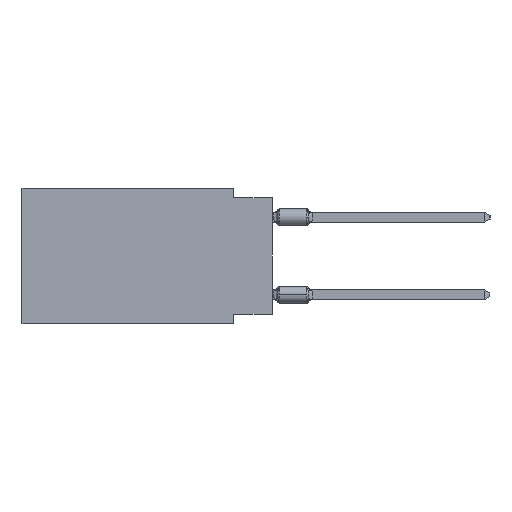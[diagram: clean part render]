
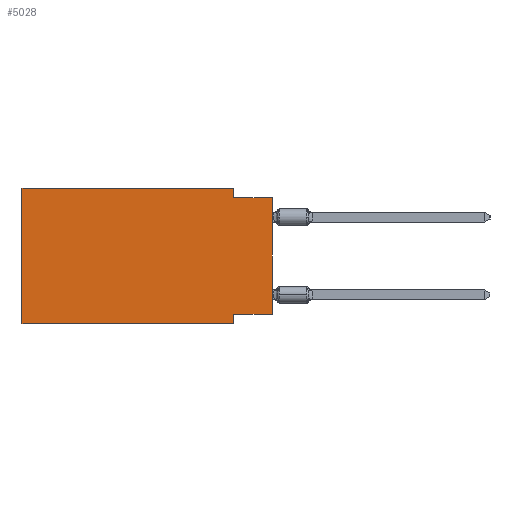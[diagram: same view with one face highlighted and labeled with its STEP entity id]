
A CAD part, left-side view. The second image highlights one B-rep face of the part: STEP entity #5028.
In plain terms, the highlighted planar face has unit normal (-1, 0, 0).
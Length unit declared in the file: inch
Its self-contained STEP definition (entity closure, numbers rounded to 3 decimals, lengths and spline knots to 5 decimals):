
#261 = DIRECTION ( 'NONE',  ( 0., -1., 0. ) ) ;
#508 = ORIENTED_EDGE ( 'NONE', *, *, #28338, .F. ) ;
#1469 = CARTESIAN_POINT ( 'NONE',  ( 0., 0.1, 0. ) ) ;
#1849 = AXIS2_PLACEMENT_3D ( 'NONE', #16052, #23807, #29257 ) ;
#3038 = ORIENTED_EDGE ( 'NONE', *, *, #13837, .T. ) ;
#3196 = LINE ( 'NONE', #21132, #12937 ) ;
#3567 = DIRECTION ( 'NONE',  ( 0., 0., 1. ) ) ;
#3634 = VECTOR ( 'NONE', #3567, 39.37008 ) ;
#4015 = VERTEX_POINT ( 'NONE', #17050 ) ;
#4470 = VECTOR ( 'NONE', #19000, 39.37008 ) ;
#4859 = VECTOR ( 'NONE', #8690, 39.37008 ) ;
#5028 = ADVANCED_FACE ( 'NONE', ( #29084 ), #23972, .F. ) ;
#5679 = CARTESIAN_POINT ( 'NONE',  ( 0., 0.645, -0.35 ) ) ;
#6104 = CARTESIAN_POINT ( 'NONE',  ( 0., 0.1, -0.35 ) ) ;
#7061 = EDGE_CURVE ( 'NONE', #13151, #31443, #3196, .T. ) ;
#7130 = DIRECTION ( 'NONE',  ( 0., 1., 0. ) ) ;
#7757 = EDGE_CURVE ( 'NONE', #9319, #26958, #9217, .T. ) ;
#8463 = ORIENTED_EDGE ( 'NONE', *, *, #7061, .T. ) ;
#8530 = LINE ( 'NONE', #16111, #4859 ) ;
#8581 = CARTESIAN_POINT ( 'NONE',  ( 0., 0., -0.325 ) ) ;
#8690 = DIRECTION ( 'NONE',  ( 0., -1., 0. ) ) ;
#9217 = LINE ( 'NONE', #24230, #27576 ) ;
#9319 = VERTEX_POINT ( 'NONE', #9963 ) ;
#9440 = VERTEX_POINT ( 'NONE', #15074 ) ;
#9963 = CARTESIAN_POINT ( 'NONE',  ( 0., 0.1, -0.325 ) ) ;
#10786 = LINE ( 'NONE', #5679, #29241 ) ;
#10972 = LINE ( 'NONE', #31091, #3634 ) ;
#11116 = VERTEX_POINT ( 'NONE', #1469 ) ;
#12760 = EDGE_CURVE ( 'NONE', #13151, #9319, #26919, .T. ) ;
#12937 = VECTOR ( 'NONE', #28411, 39.37008 ) ;
#13151 = VERTEX_POINT ( 'NONE', #8581 ) ;
#13837 = EDGE_CURVE ( 'NONE', #25378, #26958, #10786, .T. ) ;
#15074 = CARTESIAN_POINT ( 'NONE',  ( 0., 0.645, 0. ) ) ;
#15675 = CARTESIAN_POINT ( 'NONE',  ( 0., 0.645, -0.35 ) ) ;
#16036 = EDGE_CURVE ( 'NONE', #25378, #9440, #10972, .T. ) ;
#16052 = CARTESIAN_POINT ( 'NONE',  ( 0., 0.645, 0. ) ) ;
#16111 = CARTESIAN_POINT ( 'NONE',  ( 0., 0.645, 0. ) ) ;
#16929 = ORIENTED_EDGE ( 'NONE', *, *, #12760, .F. ) ;
#17050 = CARTESIAN_POINT ( 'NONE',  ( 0., 0.1, -0.025 ) ) ;
#18084 = ORIENTED_EDGE ( 'NONE', *, *, #7757, .F. ) ;
#18510 = LINE ( 'NONE', #31202, #4470 ) ;
#19000 = DIRECTION ( 'NONE',  ( 0., 0., -1. ) ) ;
#19529 = ORIENTED_EDGE ( 'NONE', *, *, #21622, .F. ) ;
#21132 = CARTESIAN_POINT ( 'NONE',  ( 0., 0., 0. ) ) ;
#21622 = EDGE_CURVE ( 'NONE', #9440, #11116, #8530, .T. ) ;
#21746 = DIRECTION ( 'NONE',  ( 0., 0., -1. ) ) ;
#21915 = DIRECTION ( 'NONE',  ( 0., -1., 0. ) ) ;
#23251 = LINE ( 'NONE', #26552, #27277 ) ;
#23389 = CARTESIAN_POINT ( 'NONE',  ( 0., 0., -0.025 ) ) ;
#23807 = DIRECTION ( 'NONE',  ( 1., 0., 0. ) ) ;
#23972 = PLANE ( 'NONE',  #1849 ) ;
#24029 = EDGE_CURVE ( 'NONE', #11116, #4015, #18510, .T. ) ;
#24230 = CARTESIAN_POINT ( 'NONE',  ( 0., 0.1, -0.35 ) ) ;
#25378 = VERTEX_POINT ( 'NONE', #15675 ) ;
#26140 = EDGE_LOOP ( 'NONE', ( #8463, #508, #27826, #19529, #30646, #3038, #18084, #16929 ) ) ;
#26552 = CARTESIAN_POINT ( 'NONE',  ( 0., 0., -0.025 ) ) ;
#26622 = VECTOR ( 'NONE', #7130, 39.37008 ) ;
#26919 = LINE ( 'NONE', #29402, #26622 ) ;
#26958 = VERTEX_POINT ( 'NONE', #6104 ) ;
#27277 = VECTOR ( 'NONE', #21915, 39.37008 ) ;
#27576 = VECTOR ( 'NONE', #21746, 39.37008 ) ;
#27826 = ORIENTED_EDGE ( 'NONE', *, *, #24029, .F. ) ;
#28338 = EDGE_CURVE ( 'NONE', #4015, #31443, #23251, .T. ) ;
#28411 = DIRECTION ( 'NONE',  ( 0., 0., 1. ) ) ;
#29084 = FACE_OUTER_BOUND ( 'NONE', #26140, .T. ) ;
#29241 = VECTOR ( 'NONE', #261, 39.37008 ) ;
#29257 = DIRECTION ( 'NONE',  ( 0., 0., -1. ) ) ;
#29402 = CARTESIAN_POINT ( 'NONE',  ( 0., 0., -0.325 ) ) ;
#30646 = ORIENTED_EDGE ( 'NONE', *, *, #16036, .F. ) ;
#31091 = CARTESIAN_POINT ( 'NONE',  ( 0., 0.645, 0. ) ) ;
#31202 = CARTESIAN_POINT ( 'NONE',  ( 0., 0.1, 0. ) ) ;
#31443 = VERTEX_POINT ( 'NONE', #23389 ) ;
